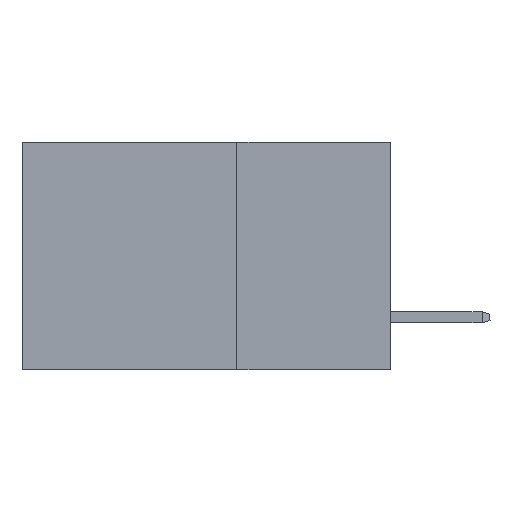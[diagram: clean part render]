
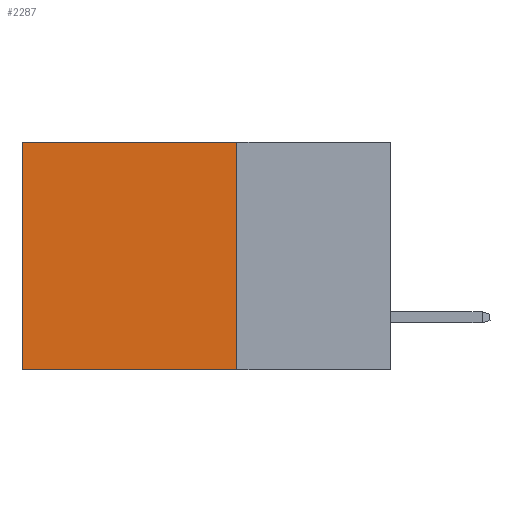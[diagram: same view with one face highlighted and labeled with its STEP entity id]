
A CAD part, left-side view. The second image highlights one B-rep face of the part: STEP entity #2287.
In plain terms, the highlighted planar face has unit normal (-1, 0, 0).
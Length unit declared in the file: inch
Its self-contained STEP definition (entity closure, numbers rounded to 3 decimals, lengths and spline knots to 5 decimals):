
#52 = VECTOR ( 'NONE', #4800, 39.37008 ) ;
#290 = DIRECTION ( 'NONE',  ( 0., 1., 0. ) ) ;
#494 = EDGE_CURVE ( 'NONE', #5269, #648, #8547, .T. ) ;
#648 = VERTEX_POINT ( 'NONE', #1928 ) ;
#993 = ORIENTED_EDGE ( 'NONE', *, *, #5570, .T. ) ;
#1029 = LINE ( 'NONE', #4827, #52 ) ;
#1632 = DIRECTION ( 'NONE',  ( 0., 0., -1. ) ) ;
#1928 = CARTESIAN_POINT ( 'NONE',  ( 0.2875, 0.6, 0. ) ) ;
#2117 = LINE ( 'NONE', #2713, #3782 ) ;
#2287 = ADVANCED_FACE ( 'NONE', ( #2385 ), #2864, .F. ) ;
#2385 = FACE_OUTER_BOUND ( 'NONE', #6925, .T. ) ;
#2394 = CARTESIAN_POINT ( 'NONE',  ( 0.2875, 0.6, 0. ) ) ;
#2402 = VECTOR ( 'NONE', #290, 39.37008 ) ;
#2713 = CARTESIAN_POINT ( 'NONE',  ( 0.2875, 0.25, -0.37 ) ) ;
#2784 = ORIENTED_EDGE ( 'NONE', *, *, #3655, .F. ) ;
#2864 = PLANE ( 'NONE',  #6839 ) ;
#3491 = DIRECTION ( 'NONE',  ( 0., 1., 0. ) ) ;
#3655 = EDGE_CURVE ( 'NONE', #4304, #8329, #2117, .T. ) ;
#3678 = CARTESIAN_POINT ( 'NONE',  ( 0.2875, 0.25, 0. ) ) ;
#3782 = VECTOR ( 'NONE', #3491, 39.37008 ) ;
#4304 = VERTEX_POINT ( 'NONE', #6373 ) ;
#4399 = DIRECTION ( 'NONE',  ( 0., 0., -1. ) ) ;
#4800 = DIRECTION ( 'NONE',  ( 0., 0., -1. ) ) ;
#4827 = CARTESIAN_POINT ( 'NONE',  ( 0.2875, 0.25, 0. ) ) ;
#5269 = VERTEX_POINT ( 'NONE', #3678 ) ;
#5570 = EDGE_CURVE ( 'NONE', #648, #8329, #9697, .T. ) ;
#6140 = CARTESIAN_POINT ( 'NONE',  ( 0.2875, 0.6, -0.37 ) ) ;
#6373 = CARTESIAN_POINT ( 'NONE',  ( 0.2875, 0.25, -0.37 ) ) ;
#6839 = AXIS2_PLACEMENT_3D ( 'NONE', #9043, #8978, #4399 ) ;
#6925 = EDGE_LOOP ( 'NONE', ( #993, #2784, #9640, #7963 ) ) ;
#7963 = ORIENTED_EDGE ( 'NONE', *, *, #494, .T. ) ;
#8329 = VERTEX_POINT ( 'NONE', #6140 ) ;
#8547 = LINE ( 'NONE', #8742, #2402 ) ;
#8742 = CARTESIAN_POINT ( 'NONE',  ( 0.2875, 0.25, 0. ) ) ;
#8830 = VECTOR ( 'NONE', #1632, 39.37008 ) ;
#8978 = DIRECTION ( 'NONE',  ( 1., 0., 0. ) ) ;
#9043 = CARTESIAN_POINT ( 'NONE',  ( 0.2875, 0.25, 0. ) ) ;
#9640 = ORIENTED_EDGE ( 'NONE', *, *, #9871, .F. ) ;
#9697 = LINE ( 'NONE', #2394, #8830 ) ;
#9871 = EDGE_CURVE ( 'NONE', #5269, #4304, #1029, .T. ) ;
